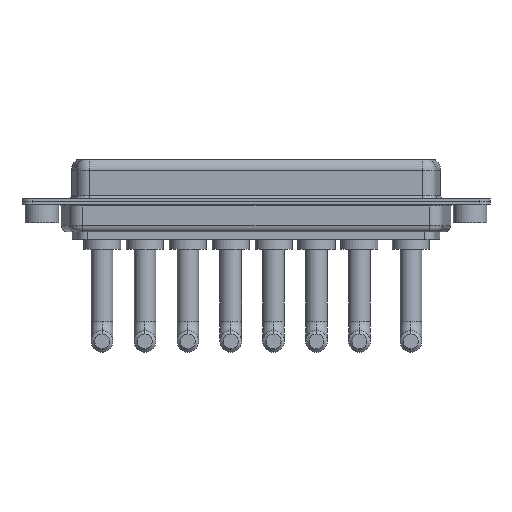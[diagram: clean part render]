
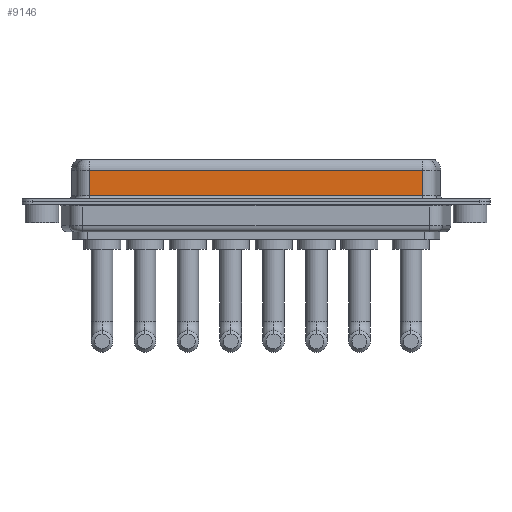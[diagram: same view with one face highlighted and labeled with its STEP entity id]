
A CAD part, front view. The second image highlights one B-rep face of the part: STEP entity #9146.
In plain terms, the highlighted planar face has unit normal (0, -1, 0).
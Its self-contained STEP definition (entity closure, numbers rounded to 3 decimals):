
#114 = LINE ( 'NONE', #7197, #486 ) ;
#486 = VECTOR ( 'NONE', #3081, 1000. ) ;
#775 = VERTEX_POINT ( 'NONE', #4108 ) ;
#938 = VECTOR ( 'NONE', #12803, 1000. ) ;
#1043 = ORIENTED_EDGE ( 'NONE', *, *, #9048, .T. ) ;
#1403 = CARTESIAN_POINT ( 'NONE',  ( 7.038, -3.95, 0.9 ) ) ;
#1719 = LINE ( 'NONE', #9847, #9365 ) ;
#2231 = EDGE_LOOP ( 'NONE', ( #11787, #1043, #12730, #13011 ) ) ;
#2631 = VERTEX_POINT ( 'NONE', #3047 ) ;
#2836 = DIRECTION ( 'NONE',  ( 0., 0., -1. ) ) ;
#2892 = FACE_OUTER_BOUND ( 'NONE', #2231, .T. ) ;
#3047 = CARTESIAN_POINT ( 'NONE',  ( 56.462, -3.95, 4.65 ) ) ;
#3081 = DIRECTION ( 'NONE',  ( 1., 0., 0. ) ) ;
#3178 = EDGE_CURVE ( 'NONE', #2631, #12964, #12003, .T. ) ;
#4108 = CARTESIAN_POINT ( 'NONE',  ( 7.038, -3.95, 4.65 ) ) ;
#4757 = DIRECTION ( 'NONE',  ( 0., 0., -1. ) ) ;
#5037 = AXIS2_PLACEMENT_3D ( 'NONE', #5721, #11843, #6795 ) ;
#5721 = CARTESIAN_POINT ( 'NONE',  ( 56.462, -3.95, 6.4 ) ) ;
#6007 = VERTEX_POINT ( 'NONE', #1403 ) ;
#6795 = DIRECTION ( 'NONE',  ( 0., 0., 1. ) ) ;
#7197 = CARTESIAN_POINT ( 'NONE',  ( 56.462, -3.95, 0.9 ) ) ;
#8324 = CARTESIAN_POINT ( 'NONE',  ( 56.462, -3.95, 6.4 ) ) ;
#8623 = EDGE_CURVE ( 'NONE', #6007, #12964, #114, .T. ) ;
#8742 = CARTESIAN_POINT ( 'NONE',  ( 56.462, -3.95, 4.65 ) ) ;
#9048 = EDGE_CURVE ( 'NONE', #2631, #775, #11591, .T. ) ;
#9146 = ADVANCED_FACE ( 'NONE', ( #2892 ), #13004, .F. ) ;
#9365 = VECTOR ( 'NONE', #4757, 1000. ) ;
#9847 = CARTESIAN_POINT ( 'NONE',  ( 7.038, -3.95, 6.4 ) ) ;
#11128 = EDGE_CURVE ( 'NONE', #775, #6007, #1719, .T. ) ;
#11591 = LINE ( 'NONE', #8742, #938 ) ;
#11689 = VECTOR ( 'NONE', #2836, 1000. ) ;
#11787 = ORIENTED_EDGE ( 'NONE', *, *, #3178, .F. ) ;
#11843 = DIRECTION ( 'NONE',  ( 0., 1., 0. ) ) ;
#12003 = LINE ( 'NONE', #8324, #11689 ) ;
#12730 = ORIENTED_EDGE ( 'NONE', *, *, #11128, .T. ) ;
#12803 = DIRECTION ( 'NONE',  ( -1., 0., 0. ) ) ;
#12864 = CARTESIAN_POINT ( 'NONE',  ( 56.462, -3.95, 0.9 ) ) ;
#12964 = VERTEX_POINT ( 'NONE', #12864 ) ;
#13004 = PLANE ( 'NONE',  #5037 ) ;
#13011 = ORIENTED_EDGE ( 'NONE', *, *, #8623, .T. ) ;
